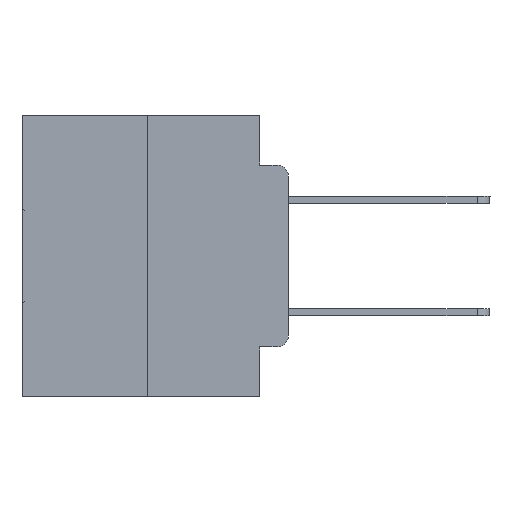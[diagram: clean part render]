
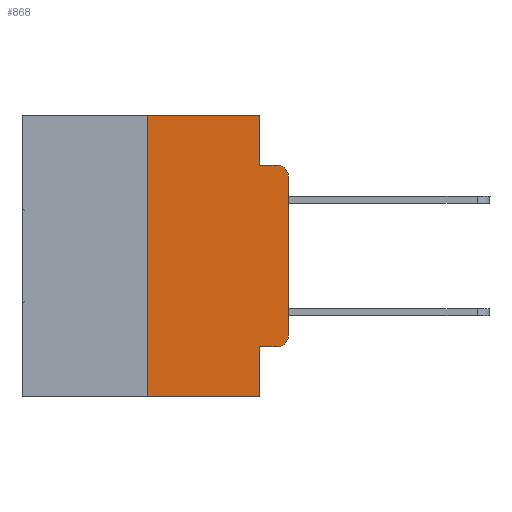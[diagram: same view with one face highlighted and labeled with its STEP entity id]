
A CAD part, left-side view. The second image highlights one B-rep face of the part: STEP entity #868.
In plain terms, the highlighted planar face has unit normal (-1, 0, 0).
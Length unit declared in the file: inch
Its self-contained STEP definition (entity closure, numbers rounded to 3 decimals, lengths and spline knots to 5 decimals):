
#176 = VERTEX_POINT ( 'NONE', #5306 ) ;
#635 = EDGE_CURVE ( 'NONE', #26751, #7720, #8336, .T. ) ;
#868 = ADVANCED_FACE ( 'NONE', ( #18831 ), #25432, .F. ) ;
#1264 = EDGE_CURVE ( 'NONE', #20568, #176, #21665, .T. ) ;
#1641 = VECTOR ( 'NONE', #29034, 39.37008 ) ;
#1705 = CARTESIAN_POINT ( 'NONE',  ( 0., 0.051, -0.4115 ) ) ;
#1732 = LINE ( 'NONE', #14977, #7958 ) ;
#2867 = DIRECTION ( 'NONE',  ( 0., 0., -1. ) ) ;
#3175 = CARTESIAN_POINT ( 'NONE',  ( 0., 0.051, 0. ) ) ;
#3542 = CARTESIAN_POINT ( 'NONE',  ( 0., 0.051, -0.0885 ) ) ;
#3683 = CARTESIAN_POINT ( 'NONE',  ( 0., 0.051, 0. ) ) ;
#4070 = VERTEX_POINT ( 'NONE', #20219 ) ;
#4796 = EDGE_CURVE ( 'NONE', #11432, #18034, #10659, .T. ) ;
#4847 = LINE ( 'NONE', #20106, #9638 ) ;
#5306 = CARTESIAN_POINT ( 'NONE',  ( 0., 0.25, 0. ) ) ;
#5610 = CIRCLE ( 'NONE', #28279, 0.02 ) ;
#6684 = ORIENTED_EDGE ( 'NONE', *, *, #10092, .T. ) ;
#7409 = ORIENTED_EDGE ( 'NONE', *, *, #15916, .T. ) ;
#7720 = VERTEX_POINT ( 'NONE', #7726 ) ;
#7726 = CARTESIAN_POINT ( 'NONE',  ( 0., 0.02, -0.4115 ) ) ;
#7958 = VECTOR ( 'NONE', #26435, 39.37008 ) ;
#8336 = LINE ( 'NONE', #22454, #18485 ) ;
#9078 = CARTESIAN_POINT ( 'NONE',  ( 0., 0.051, 0. ) ) ;
#9291 = VERTEX_POINT ( 'NONE', #26824 ) ;
#9417 = VECTOR ( 'NONE', #14015, 39.37008 ) ;
#9638 = VECTOR ( 'NONE', #10976, 39.37008 ) ;
#9658 = ORIENTED_EDGE ( 'NONE', *, *, #4796, .F. ) ;
#9767 = CARTESIAN_POINT ( 'NONE',  ( 0., 0.02, -0.3915 ) ) ;
#10092 = EDGE_CURVE ( 'NONE', #26009, #17139, #30012, .T. ) ;
#10659 = LINE ( 'NONE', #3175, #22172 ) ;
#10976 = DIRECTION ( 'NONE',  ( 0., -1., 0. ) ) ;
#11432 = VERTEX_POINT ( 'NONE', #9078 ) ;
#11732 = VECTOR ( 'NONE', #17759, 39.37008 ) ;
#11848 = ORIENTED_EDGE ( 'NONE', *, *, #635, .T. ) ;
#12084 = DIRECTION ( 'NONE',  ( 0., 0., -1. ) ) ;
#12246 = EDGE_CURVE ( 'NONE', #7720, #26009, #5610, .T. ) ;
#12580 = CARTESIAN_POINT ( 'NONE',  ( 0., 0., -0.3915 ) ) ;
#13110 = CARTESIAN_POINT ( 'NONE',  ( 0., 0., 0. ) ) ;
#13181 = CARTESIAN_POINT ( 'NONE',  ( 0., 0.02, -0.1085 ) ) ;
#13314 = CARTESIAN_POINT ( 'NONE',  ( 0., 0., -0.1085 ) ) ;
#13338 = LINE ( 'NONE', #3683, #1641 ) ;
#14015 = DIRECTION ( 'NONE',  ( 0., 0., 1. ) ) ;
#14173 = CARTESIAN_POINT ( 'NONE',  ( 0., 0.051, -0.0885 ) ) ;
#14312 = CARTESIAN_POINT ( 'NONE',  ( 0., 0.25, 0. ) ) ;
#14977 = CARTESIAN_POINT ( 'NONE',  ( 0., 0.473, -0.5 ) ) ;
#15100 = AXIS2_PLACEMENT_3D ( 'NONE', #13181, #29235, #15497 ) ;
#15497 = DIRECTION ( 'NONE',  ( 0., 0., -1. ) ) ;
#15575 = CIRCLE ( 'NONE', #15100, 0.02 ) ;
#15795 = ORIENTED_EDGE ( 'NONE', *, *, #21988, .F. ) ;
#15916 = EDGE_CURVE ( 'NONE', #17139, #4070, #15575, .T. ) ;
#17139 = VERTEX_POINT ( 'NONE', #13314 ) ;
#17330 = CARTESIAN_POINT ( 'NONE',  ( 0., 0.25, -0.5 ) ) ;
#17759 = DIRECTION ( 'NONE',  ( 0., 0., 1. ) ) ;
#18034 = VERTEX_POINT ( 'NONE', #14173 ) ;
#18485 = VECTOR ( 'NONE', #22151, 39.37008 ) ;
#18544 = AXIS2_PLACEMENT_3D ( 'NONE', #26143, #25981, #20796 ) ;
#18831 = FACE_OUTER_BOUND ( 'NONE', #20149, .T. ) ;
#19277 = EDGE_CURVE ( 'NONE', #20568, #9291, #1732, .T. ) ;
#20106 = CARTESIAN_POINT ( 'NONE',  ( 0., 0.473, 0. ) ) ;
#20149 = EDGE_LOOP ( 'NONE', ( #6684, #7409, #26583, #9658, #15795, #21903, #29433, #24049, #11848, #25509 ) ) ;
#20219 = CARTESIAN_POINT ( 'NONE',  ( 0., 0.02, -0.0885 ) ) ;
#20568 = VERTEX_POINT ( 'NONE', #17330 ) ;
#20796 = DIRECTION ( 'NONE',  ( 0., 0., -1. ) ) ;
#21092 = VECTOR ( 'NONE', #26736, 39.37008 ) ;
#21665 = LINE ( 'NONE', #14312, #9417 ) ;
#21903 = ORIENTED_EDGE ( 'NONE', *, *, #1264, .F. ) ;
#21988 = EDGE_CURVE ( 'NONE', #176, #11432, #4847, .T. ) ;
#22151 = DIRECTION ( 'NONE',  ( 0., -1., 0. ) ) ;
#22172 = VECTOR ( 'NONE', #2867, 39.37008 ) ;
#22454 = CARTESIAN_POINT ( 'NONE',  ( 0., 0.051, -0.4115 ) ) ;
#24049 = ORIENTED_EDGE ( 'NONE', *, *, #26127, .F. ) ;
#25432 = PLANE ( 'NONE',  #18544 ) ;
#25509 = ORIENTED_EDGE ( 'NONE', *, *, #12246, .T. ) ;
#25867 = DIRECTION ( 'NONE',  ( -1., 0., 0. ) ) ;
#25981 = DIRECTION ( 'NONE',  ( 1., 0., 0. ) ) ;
#26009 = VERTEX_POINT ( 'NONE', #12580 ) ;
#26127 = EDGE_CURVE ( 'NONE', #26751, #9291, #13338, .T. ) ;
#26143 = CARTESIAN_POINT ( 'NONE',  ( 0., 0.473, 0. ) ) ;
#26435 = DIRECTION ( 'NONE',  ( 0., -1., 0. ) ) ;
#26583 = ORIENTED_EDGE ( 'NONE', *, *, #28475, .F. ) ;
#26736 = DIRECTION ( 'NONE',  ( 0., -1., 0. ) ) ;
#26751 = VERTEX_POINT ( 'NONE', #1705 ) ;
#26824 = CARTESIAN_POINT ( 'NONE',  ( 0., 0.051, -0.5 ) ) ;
#27237 = LINE ( 'NONE', #3542, #21092 ) ;
#28279 = AXIS2_PLACEMENT_3D ( 'NONE', #9767, #25867, #12084 ) ;
#28475 = EDGE_CURVE ( 'NONE', #18034, #4070, #27237, .T. ) ;
#29034 = DIRECTION ( 'NONE',  ( 0., 0., -1. ) ) ;
#29235 = DIRECTION ( 'NONE',  ( -1., 0., 0. ) ) ;
#29433 = ORIENTED_EDGE ( 'NONE', *, *, #19277, .T. ) ;
#30012 = LINE ( 'NONE', #13110, #11732 ) ;
